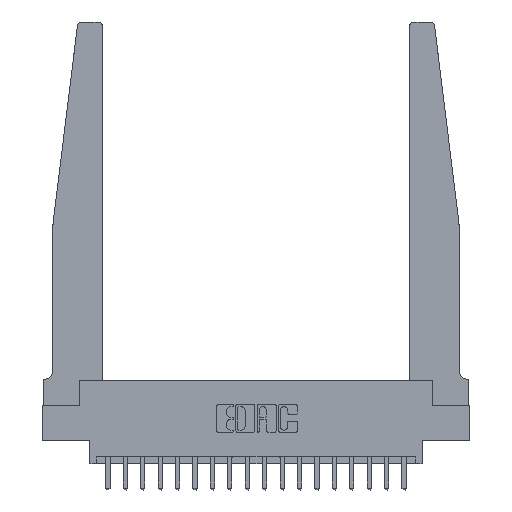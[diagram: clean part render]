
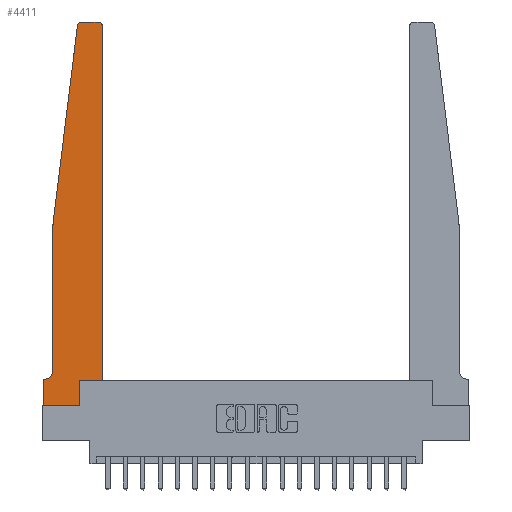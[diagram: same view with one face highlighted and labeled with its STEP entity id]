
A CAD part, top view. The second image highlights one B-rep face of the part: STEP entity #4411.
In plain terms, the highlighted planar face has unit normal (0, 0, 1).
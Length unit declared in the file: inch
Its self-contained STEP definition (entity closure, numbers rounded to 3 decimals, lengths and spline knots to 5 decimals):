
#22 = DIRECTION ( 'NONE',  ( 1., 0., 0. ) ) ;
#227 = VERTEX_POINT ( 'NONE', #2156 ) ;
#364 = DIRECTION ( 'NONE',  ( -1., 0., 0. ) ) ;
#458 = LINE ( 'NONE', #6808, #3297 ) ;
#664 = DIRECTION ( 'NONE',  ( 1., 0., 0. ) ) ;
#807 = VECTOR ( 'NONE', #15924, 39.37008 ) ;
#1424 = CARTESIAN_POINT ( 'NONE',  ( 0., 0., 0.37 ) ) ;
#1425 = AXIS2_PLACEMENT_3D ( 'NONE', #7610, #13911, #15346 ) ;
#1429 = VERTEX_POINT ( 'NONE', #12131 ) ;
#1484 = VERTEX_POINT ( 'NONE', #5818 ) ;
#1936 = LINE ( 'NONE', #17851, #13705 ) ;
#2156 = CARTESIAN_POINT ( 'NONE',  ( 0.2605, 0.18, 0.37 ) ) ;
#2558 = VERTEX_POINT ( 'NONE', #7941 ) ;
#3171 = CARTESIAN_POINT ( 'NONE',  ( 0.015, 0.2375, 0.37 ) ) ;
#3297 = VECTOR ( 'NONE', #9694, 39.37008 ) ;
#3329 = CARTESIAN_POINT ( 'NONE',  ( 0.27653, 2.72, 0.37 ) ) ;
#3415 = DIRECTION ( 'NONE',  ( 1., 0., 0. ) ) ;
#3453 = CARTESIAN_POINT ( 'NONE',  ( 0.2605, 0., 0.37 ) ) ;
#3644 = EDGE_CURVE ( 'NONE', #14918, #2558, #16607, .T. ) ;
#3781 = CARTESIAN_POINT ( 'NONE',  ( 0.425, 0.18, 0.37 ) ) ;
#3981 = ORIENTED_EDGE ( 'NONE', *, *, #13576, .T. ) ;
#4034 = VECTOR ( 'NONE', #664, 39.37008 ) ;
#4411 = ADVANCED_FACE ( 'NONE', ( #5097 ), #8098, .T. ) ;
#4690 = EDGE_CURVE ( 'NONE', #7104, #1429, #6131, .T. ) ;
#4746 = VERTEX_POINT ( 'NONE', #10969 ) ;
#5085 = CARTESIAN_POINT ( 'NONE',  ( 0., 0., 0.37 ) ) ;
#5097 = FACE_OUTER_BOUND ( 'NONE', #19852, .T. ) ;
#5118 = DIRECTION ( 'NONE',  ( 1., 0., 0. ) ) ;
#5439 = ORIENTED_EDGE ( 'NONE', *, *, #12789, .T. ) ;
#5796 = EDGE_CURVE ( 'NONE', #8373, #4746, #13660, .T. ) ;
#5818 = CARTESIAN_POINT ( 'NONE',  ( 0.425, 0.18, 0.37 ) ) ;
#6052 = ORIENTED_EDGE ( 'NONE', *, *, #4690, .T. ) ;
#6131 = CIRCLE ( 'NONE', #12733, 0.05 ) ;
#6154 = VERTEX_POINT ( 'NONE', #18255 ) ;
#6512 = EDGE_CURVE ( 'NONE', #2558, #6154, #458, .T. ) ;
#6542 = EDGE_CURVE ( 'NONE', #4746, #7104, #11670, .T. ) ;
#6620 = ORIENTED_EDGE ( 'NONE', *, *, #10128, .T. ) ;
#6808 = CARTESIAN_POINT ( 'NONE',  ( 0.25, 2.75, 0.37 ) ) ;
#7104 = VERTEX_POINT ( 'NONE', #13663 ) ;
#7610 = CARTESIAN_POINT ( 'NONE',  ( 0.395, 2.72, 0.37 ) ) ;
#7762 = DIRECTION ( 'NONE',  ( 0., -1., 0. ) ) ;
#7941 = CARTESIAN_POINT ( 'NONE',  ( 0.395, 2.75, 0.37 ) ) ;
#8098 = PLANE ( 'NONE',  #14685 ) ;
#8357 = LINE ( 'NONE', #3781, #4034 ) ;
#8373 = VERTEX_POINT ( 'NONE', #16217 ) ;
#9172 = CIRCLE ( 'NONE', #20395, 0.03 ) ;
#9679 = ORIENTED_EDGE ( 'NONE', *, *, #15219, .T. ) ;
#9693 = EDGE_CURVE ( 'NONE', #1484, #14918, #1936, .T. ) ;
#9694 = DIRECTION ( 'NONE',  ( -1., 0., 0. ) ) ;
#10036 = ORIENTED_EDGE ( 'NONE', *, *, #6512, .T. ) ;
#10128 = EDGE_CURVE ( 'NONE', #227, #1484, #8357, .T. ) ;
#10571 = CARTESIAN_POINT ( 'NONE',  ( 0., 0.1875, 0.37 ) ) ;
#10907 = VECTOR ( 'NONE', #16292, 39.37008 ) ;
#10969 = CARTESIAN_POINT ( 'NONE',  ( 0.065, 1.25, 0.37 ) ) ;
#11670 = LINE ( 'NONE', #17818, #10907 ) ;
#12019 = CARTESIAN_POINT ( 'NONE',  ( 0.065, 1.25, 0.37 ) ) ;
#12131 = CARTESIAN_POINT ( 'NONE',  ( 0.015, 0.1875, 0.37 ) ) ;
#12370 = VERTEX_POINT ( 'NONE', #5085 ) ;
#12733 = AXIS2_PLACEMENT_3D ( 'NONE', #3171, #14063, #17029 ) ;
#12789 = EDGE_CURVE ( 'NONE', #1429, #13255, #17724, .T. ) ;
#12843 = LINE ( 'NONE', #16120, #807 ) ;
#12984 = LINE ( 'NONE', #19253, #19399 ) ;
#13037 = ORIENTED_EDGE ( 'NONE', *, *, #14887, .T. ) ;
#13255 = VERTEX_POINT ( 'NONE', #10571 ) ;
#13337 = DIRECTION ( 'NONE',  ( 0., 1., 0. ) ) ;
#13576 = EDGE_CURVE ( 'NONE', #16943, #227, #12843, .T. ) ;
#13660 = LINE ( 'NONE', #12019, #17781 ) ;
#13663 = CARTESIAN_POINT ( 'NONE',  ( 0.065, 0.2375, 0.37 ) ) ;
#13705 = VECTOR ( 'NONE', #13337, 39.37008 ) ;
#13911 = DIRECTION ( 'NONE',  ( 0., 0., 1. ) ) ;
#14063 = DIRECTION ( 'NONE',  ( 0., 0., -1. ) ) ;
#14685 = AXIS2_PLACEMENT_3D ( 'NONE', #14686, #17659, #3415 ) ;
#14686 = CARTESIAN_POINT ( 'NONE',  ( 0., 0.1875, 0.37 ) ) ;
#14835 = EDGE_CURVE ( 'NONE', #6154, #8373, #9172, .T. ) ;
#14887 = EDGE_CURVE ( 'NONE', #12370, #16943, #12984, .T. ) ;
#14918 = VERTEX_POINT ( 'NONE', #17786 ) ;
#15203 = ORIENTED_EDGE ( 'NONE', *, *, #9693, .T. ) ;
#15219 = EDGE_CURVE ( 'NONE', #13255, #12370, #15602, .T. ) ;
#15346 = DIRECTION ( 'NONE',  ( 1., 0., 0. ) ) ;
#15602 = LINE ( 'NONE', #1424, #19708 ) ;
#15924 = DIRECTION ( 'NONE',  ( 0., 1., 0. ) ) ;
#16120 = CARTESIAN_POINT ( 'NONE',  ( 0.2605, 0.18, 0.37 ) ) ;
#16217 = CARTESIAN_POINT ( 'NONE',  ( 0.24675, 2.72367, 0.37 ) ) ;
#16287 = ORIENTED_EDGE ( 'NONE', *, *, #5796, .T. ) ;
#16292 = DIRECTION ( 'NONE',  ( 0., -1., 0. ) ) ;
#16428 = VECTOR ( 'NONE', #364, 39.37008 ) ;
#16607 = CIRCLE ( 'NONE', #1425, 0.03 ) ;
#16672 = ORIENTED_EDGE ( 'NONE', *, *, #14835, .T. ) ;
#16943 = VERTEX_POINT ( 'NONE', #3453 ) ;
#17029 = DIRECTION ( 'NONE',  ( -1., 0., 0. ) ) ;
#17589 = DIRECTION ( 'NONE',  ( 0., 0., 1. ) ) ;
#17659 = DIRECTION ( 'NONE',  ( 0., 0., 1. ) ) ;
#17714 = ORIENTED_EDGE ( 'NONE', *, *, #3644, .T. ) ;
#17724 = LINE ( 'NONE', #19188, #16428 ) ;
#17781 = VECTOR ( 'NONE', #19716, 39.37008 ) ;
#17786 = CARTESIAN_POINT ( 'NONE',  ( 0.425, 2.72, 0.37 ) ) ;
#17818 = CARTESIAN_POINT ( 'NONE',  ( 0.065, 1.25, 0.37 ) ) ;
#17851 = CARTESIAN_POINT ( 'NONE',  ( 0.425, 0.18, 0.37 ) ) ;
#18255 = CARTESIAN_POINT ( 'NONE',  ( 0.27653, 2.75, 0.37 ) ) ;
#19188 = CARTESIAN_POINT ( 'NONE',  ( 0.065, 0.1875, 0.37 ) ) ;
#19253 = CARTESIAN_POINT ( 'NONE',  ( 0., 0., 0.37 ) ) ;
#19399 = VECTOR ( 'NONE', #5118, 39.37008 ) ;
#19651 = ORIENTED_EDGE ( 'NONE', *, *, #6542, .T. ) ;
#19708 = VECTOR ( 'NONE', #7762, 39.37008 ) ;
#19716 = DIRECTION ( 'NONE',  ( -0.122, -0.992, 0. ) ) ;
#19852 = EDGE_LOOP ( 'NONE', ( #10036, #16672, #16287, #19651, #6052, #5439, #9679, #13037, #3981, #6620, #15203, #17714 ) ) ;
#20395 = AXIS2_PLACEMENT_3D ( 'NONE', #3329, #17589, #22 ) ;
